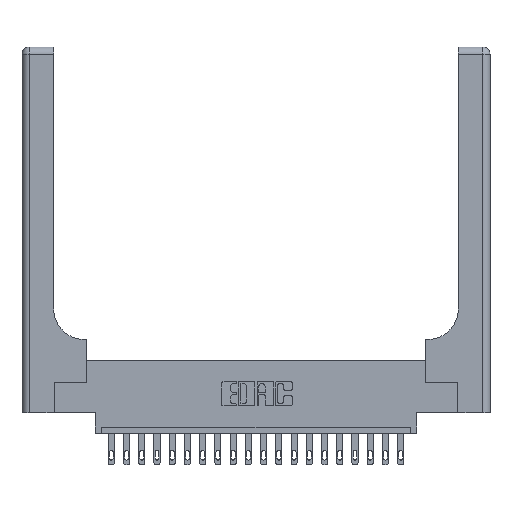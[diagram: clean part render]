
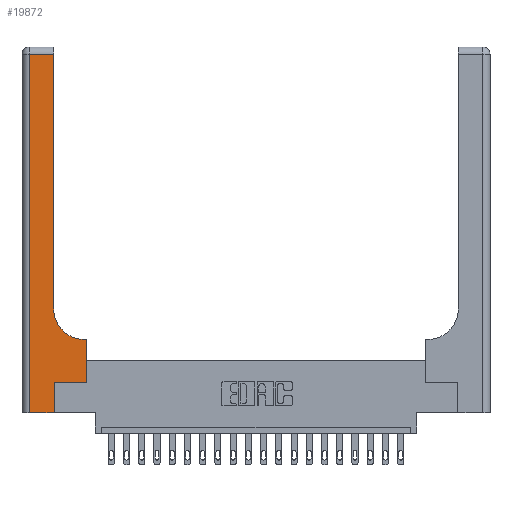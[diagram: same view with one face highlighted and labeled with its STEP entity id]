
A CAD part, top view. The second image highlights one B-rep face of the part: STEP entity #19872.
In plain terms, the highlighted planar face has unit normal (0, 0, 1).
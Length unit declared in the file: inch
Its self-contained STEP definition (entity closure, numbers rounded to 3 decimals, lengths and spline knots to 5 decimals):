
#21 = VERTEX_POINT ( 'NONE', #7636 ) ;
#569 = LINE ( 'NONE', #2588, #4651 ) ;
#947 = DIRECTION ( 'NONE',  ( 1., 0., 0. ) ) ;
#1003 = EDGE_CURVE ( 'NONE', #8961, #7658, #14256, .T. ) ;
#1129 = LINE ( 'NONE', #14305, #4694 ) ;
#1130 = CARTESIAN_POINT ( 'NONE',  ( 0., 3., 0.37 ) ) ;
#1226 = ORIENTED_EDGE ( 'NONE', *, *, #7571, .T. ) ;
#1639 = DIRECTION ( 'NONE',  ( 1., 0., 0. ) ) ;
#1876 = CARTESIAN_POINT ( 'NONE',  ( 0.528, 0.25, 0.37 ) ) ;
#1956 = CARTESIAN_POINT ( 'NONE',  ( 0.26, 0.6, 0.37 ) ) ;
#2327 = ORIENTED_EDGE ( 'NONE', *, *, #17061, .T. ) ;
#2486 = VERTEX_POINT ( 'NONE', #2878 ) ;
#2530 = ORIENTED_EDGE ( 'NONE', *, *, #12121, .T. ) ;
#2588 = CARTESIAN_POINT ( 'NONE',  ( 0.26, 3., 0.37 ) ) ;
#2698 = VECTOR ( 'NONE', #15276, 39.37008 ) ;
#2878 = CARTESIAN_POINT ( 'NONE',  ( 0.265, 0.25, 0.37 ) ) ;
#2963 = VERTEX_POINT ( 'NONE', #11450 ) ;
#3365 = DIRECTION ( 'NONE',  ( 0., 1., 0. ) ) ;
#4061 = ORIENTED_EDGE ( 'NONE', *, *, #19681, .T. ) ;
#4123 = VECTOR ( 'NONE', #17322, 39.37008 ) ;
#4465 = CARTESIAN_POINT ( 'NONE',  ( 0., 0., 0.37 ) ) ;
#4577 = AXIS2_PLACEMENT_3D ( 'NONE', #10515, #9112, #947 ) ;
#4651 = VECTOR ( 'NONE', #16850, 39.37008 ) ;
#4694 = VECTOR ( 'NONE', #7585, 39.37008 ) ;
#4823 = VECTOR ( 'NONE', #3365, 39.37008 ) ;
#5220 = EDGE_CURVE ( 'NONE', #2486, #2963, #15113, .T. ) ;
#5889 = CARTESIAN_POINT ( 'NONE',  ( 0.265, 0., 0.37 ) ) ;
#6523 = EDGE_LOOP ( 'NONE', ( #1226, #11721, #2530, #20419, #6633, #11696, #4061, #15436, #2327 ) ) ;
#6633 = ORIENTED_EDGE ( 'NONE', *, *, #13414, .T. ) ;
#7571 = EDGE_CURVE ( 'NONE', #7962, #10532, #569, .T. ) ;
#7585 = DIRECTION ( 'NONE',  ( -1., 0., 0. ) ) ;
#7636 = CARTESIAN_POINT ( 'NONE',  ( 0.06, 2.94, 0.37 ) ) ;
#7658 = VERTEX_POINT ( 'NONE', #5889 ) ;
#7962 = VERTEX_POINT ( 'NONE', #13270 ) ;
#8798 = VERTEX_POINT ( 'NONE', #10309 ) ;
#8961 = VERTEX_POINT ( 'NONE', #10957 ) ;
#9112 = DIRECTION ( 'NONE',  ( 0., 0., -1. ) ) ;
#9300 = EDGE_CURVE ( 'NONE', #10532, #21, #1129, .T. ) ;
#9694 = CARTESIAN_POINT ( 'NONE',  ( 0.265, 0.25, 0.37 ) ) ;
#10122 = DIRECTION ( 'NONE',  ( -1., 0., 0. ) ) ;
#10309 = CARTESIAN_POINT ( 'NONE',  ( 0.51, 0.6, 0.37 ) ) ;
#10515 = CARTESIAN_POINT ( 'NONE',  ( 0.51, 0.85, 0.37 ) ) ;
#10532 = VERTEX_POINT ( 'NONE', #17631 ) ;
#10725 = LINE ( 'NONE', #17637, #4123 ) ;
#10957 = CARTESIAN_POINT ( 'NONE',  ( 0.06, 0., 0.37 ) ) ;
#11450 = CARTESIAN_POINT ( 'NONE',  ( 0.528, 0.25, 0.37 ) ) ;
#11696 = ORIENTED_EDGE ( 'NONE', *, *, #5220, .T. ) ;
#11721 = ORIENTED_EDGE ( 'NONE', *, *, #9300, .T. ) ;
#12077 = FACE_OUTER_BOUND ( 'NONE', #6523, .T. ) ;
#12121 = EDGE_CURVE ( 'NONE', #21, #8961, #10725, .T. ) ;
#12390 = DIRECTION ( 'NONE',  ( -1., 0., 0. ) ) ;
#12559 = VECTOR ( 'NONE', #10122, 39.37008 ) ;
#12952 = CARTESIAN_POINT ( 'NONE',  ( 0.265, 0., 0.37 ) ) ;
#13270 = CARTESIAN_POINT ( 'NONE',  ( 0.26, 0.85, 0.37 ) ) ;
#13414 = EDGE_CURVE ( 'NONE', #7658, #2486, #16260, .T. ) ;
#14256 = LINE ( 'NONE', #4465, #15991 ) ;
#14305 = CARTESIAN_POINT ( 'NONE',  ( 0., 2.94, 0.37 ) ) ;
#15113 = LINE ( 'NONE', #9694, #18239 ) ;
#15276 = DIRECTION ( 'NONE',  ( 0., 1., 0. ) ) ;
#15436 = ORIENTED_EDGE ( 'NONE', *, *, #20154, .T. ) ;
#15813 = CIRCLE ( 'NONE', #4577, 0.25 ) ;
#15991 = VECTOR ( 'NONE', #17447, 39.37008 ) ;
#16260 = LINE ( 'NONE', #12952, #4823 ) ;
#16289 = AXIS2_PLACEMENT_3D ( 'NONE', #1130, #17287, #12390 ) ;
#16850 = DIRECTION ( 'NONE',  ( 0., 1., 0. ) ) ;
#16870 = LINE ( 'NONE', #1876, #2698 ) ;
#17061 = EDGE_CURVE ( 'NONE', #8798, #7962, #15813, .T. ) ;
#17183 = PLANE ( 'NONE',  #16289 ) ;
#17287 = DIRECTION ( 'NONE',  ( 0., 0., -1. ) ) ;
#17322 = DIRECTION ( 'NONE',  ( 0., -1., 0. ) ) ;
#17447 = DIRECTION ( 'NONE',  ( 1., 0., 0. ) ) ;
#17631 = CARTESIAN_POINT ( 'NONE',  ( 0.26, 2.94, 0.37 ) ) ;
#17637 = CARTESIAN_POINT ( 'NONE',  ( 0.06, 3., 0.37 ) ) ;
#18239 = VECTOR ( 'NONE', #1639, 39.37008 ) ;
#18747 = LINE ( 'NONE', #1956, #12559 ) ;
#18985 = VERTEX_POINT ( 'NONE', #19855 ) ;
#19681 = EDGE_CURVE ( 'NONE', #2963, #18985, #16870, .T. ) ;
#19855 = CARTESIAN_POINT ( 'NONE',  ( 0.528, 0.6, 0.37 ) ) ;
#19872 = ADVANCED_FACE ( 'NONE', ( #12077 ), #17183, .F. ) ;
#20154 = EDGE_CURVE ( 'NONE', #18985, #8798, #18747, .T. ) ;
#20419 = ORIENTED_EDGE ( 'NONE', *, *, #1003, .T. ) ;
